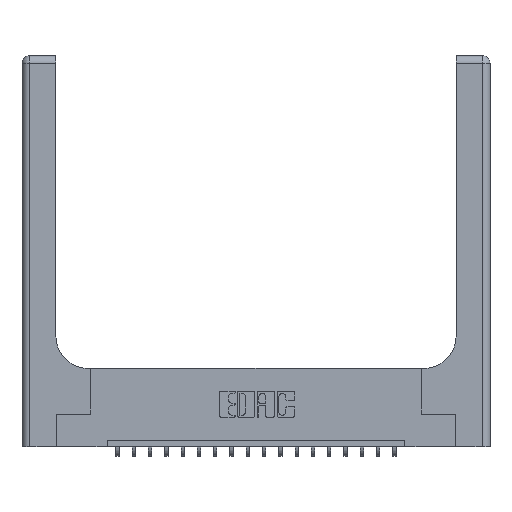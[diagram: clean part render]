
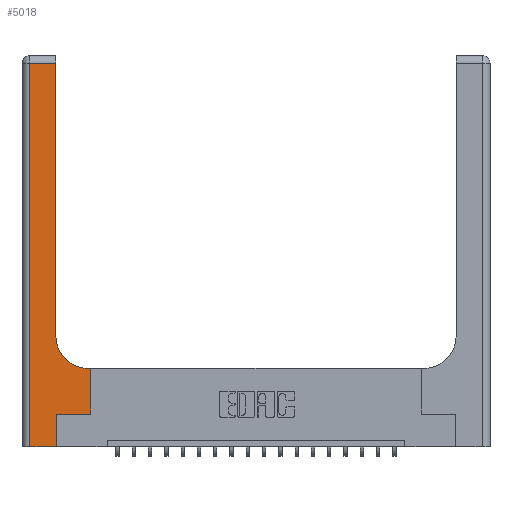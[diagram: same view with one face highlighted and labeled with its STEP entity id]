
A CAD part, top view. The second image highlights one B-rep face of the part: STEP entity #5018.
In plain terms, the highlighted planar face has unit normal (0, 0, 1).
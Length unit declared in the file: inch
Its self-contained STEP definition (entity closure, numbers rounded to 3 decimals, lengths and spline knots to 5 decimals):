
#556 = VERTEX_POINT ( 'NONE', #9216 ) ;
#884 = VERTEX_POINT ( 'NONE', #16140 ) ;
#914 = CARTESIAN_POINT ( 'NONE',  ( 0.528, 0.25, 0.37 ) ) ;
#1122 = LINE ( 'NONE', #17620, #4291 ) ;
#1272 = CARTESIAN_POINT ( 'NONE',  ( 0.51, 0.85, 0.37 ) ) ;
#1273 = ORIENTED_EDGE ( 'NONE', *, *, #6893, .T. ) ;
#1437 = CARTESIAN_POINT ( 'NONE',  ( 0.265, 0.25, 0.37 ) ) ;
#1882 = EDGE_CURVE ( 'NONE', #2824, #1946, #1122, .T. ) ;
#1936 = CARTESIAN_POINT ( 'NONE',  ( 0.265, 0., 0.37 ) ) ;
#1946 = VERTEX_POINT ( 'NONE', #18594 ) ;
#2226 = ORIENTED_EDGE ( 'NONE', *, *, #4807, .T. ) ;
#2437 = CARTESIAN_POINT ( 'NONE',  ( 0.06, 2.94, 0.37 ) ) ;
#2505 = EDGE_CURVE ( 'NONE', #884, #556, #6919, .T. ) ;
#2533 = EDGE_CURVE ( 'NONE', #2787, #11982, #18445, .T. ) ;
#2642 = ORIENTED_EDGE ( 'NONE', *, *, #5450, .T. ) ;
#2787 = VERTEX_POINT ( 'NONE', #7012 ) ;
#2809 = VECTOR ( 'NONE', #9410, 39.37008 ) ;
#2824 = VERTEX_POINT ( 'NONE', #914 ) ;
#2850 = DIRECTION ( 'NONE',  ( 1., 0., 0. ) ) ;
#2891 = DIRECTION ( 'NONE',  ( 1., 0., 0. ) ) ;
#2896 = CARTESIAN_POINT ( 'NONE',  ( 0.51, 0.6, 0.37 ) ) ;
#3967 = LINE ( 'NONE', #1936, #16065 ) ;
#4291 = VECTOR ( 'NONE', #9397, 39.37008 ) ;
#4752 = VECTOR ( 'NONE', #15321, 39.37008 ) ;
#4807 = EDGE_CURVE ( 'NONE', #12909, #2824, #18921, .T. ) ;
#4899 = ORIENTED_EDGE ( 'NONE', *, *, #2533, .T. ) ;
#4968 = PLANE ( 'NONE',  #11999 ) ;
#4972 = ORIENTED_EDGE ( 'NONE', *, *, #2505, .T. ) ;
#5018 = ADVANCED_FACE ( 'NONE', ( #14708 ), #4968, .F. ) ;
#5150 = CARTESIAN_POINT ( 'NONE',  ( 0.26, 2.94, 0.37 ) ) ;
#5159 = EDGE_CURVE ( 'NONE', #9615, #884, #5220, .T. ) ;
#5220 = LINE ( 'NONE', #10884, #4752 ) ;
#5450 = EDGE_CURVE ( 'NONE', #1946, #14128, #11665, .T. ) ;
#6278 = DIRECTION ( 'NONE',  ( 1., 0., 0. ) ) ;
#6517 = DIRECTION ( 'NONE',  ( -1., 0., 0. ) ) ;
#6765 = DIRECTION ( 'NONE',  ( -1., 0., 0. ) ) ;
#6893 = EDGE_CURVE ( 'NONE', #556, #12909, #3967, .T. ) ;
#6919 = LINE ( 'NONE', #10885, #7402 ) ;
#7012 = CARTESIAN_POINT ( 'NONE',  ( 0.26, 0.85, 0.37 ) ) ;
#7402 = VECTOR ( 'NONE', #6278, 39.37008 ) ;
#9216 = CARTESIAN_POINT ( 'NONE',  ( 0.265, 0., 0.37 ) ) ;
#9340 = CARTESIAN_POINT ( 'NONE',  ( 0.26, 3., 0.37 ) ) ;
#9397 = DIRECTION ( 'NONE',  ( 0., 1., 0. ) ) ;
#9410 = DIRECTION ( 'NONE',  ( 0., 1., 0. ) ) ;
#9615 = VERTEX_POINT ( 'NONE', #2437 ) ;
#10002 = DIRECTION ( 'NONE',  ( -1., 0., 0. ) ) ;
#10538 = CARTESIAN_POINT ( 'NONE',  ( 0.265, 0.25, 0.37 ) ) ;
#10884 = CARTESIAN_POINT ( 'NONE',  ( 0.06, 3., 0.37 ) ) ;
#10885 = CARTESIAN_POINT ( 'NONE',  ( 0., 0., 0.37 ) ) ;
#11169 = ORIENTED_EDGE ( 'NONE', *, *, #13569, .T. ) ;
#11474 = CARTESIAN_POINT ( 'NONE',  ( 0.26, 0.6, 0.37 ) ) ;
#11665 = LINE ( 'NONE', #11474, #19131 ) ;
#11691 = VECTOR ( 'NONE', #6765, 39.37008 ) ;
#11982 = VERTEX_POINT ( 'NONE', #5150 ) ;
#11999 = AXIS2_PLACEMENT_3D ( 'NONE', #18503, #15561, #6517 ) ;
#12019 = DIRECTION ( 'NONE',  ( 0., 0., -1. ) ) ;
#12652 = ORIENTED_EDGE ( 'NONE', *, *, #1882, .T. ) ;
#12909 = VERTEX_POINT ( 'NONE', #1437 ) ;
#13569 = EDGE_CURVE ( 'NONE', #14128, #2787, #15926, .T. ) ;
#14128 = VERTEX_POINT ( 'NONE', #2896 ) ;
#14708 = FACE_OUTER_BOUND ( 'NONE', #18203, .T. ) ;
#15049 = EDGE_CURVE ( 'NONE', #11982, #9615, #16143, .T. ) ;
#15292 = ORIENTED_EDGE ( 'NONE', *, *, #15049, .T. ) ;
#15321 = DIRECTION ( 'NONE',  ( 0., -1., 0. ) ) ;
#15561 = DIRECTION ( 'NONE',  ( 0., 0., -1. ) ) ;
#15926 = CIRCLE ( 'NONE', #17598, 0.25 ) ;
#16065 = VECTOR ( 'NONE', #18585, 39.37008 ) ;
#16140 = CARTESIAN_POINT ( 'NONE',  ( 0.06, 0., 0.37 ) ) ;
#16143 = LINE ( 'NONE', #17298, #11691 ) ;
#17298 = CARTESIAN_POINT ( 'NONE',  ( 0., 2.94, 0.37 ) ) ;
#17598 = AXIS2_PLACEMENT_3D ( 'NONE', #1272, #12019, #2850 ) ;
#17620 = CARTESIAN_POINT ( 'NONE',  ( 0.528, 0.25, 0.37 ) ) ;
#17996 = VECTOR ( 'NONE', #2891, 39.37008 ) ;
#18203 = EDGE_LOOP ( 'NONE', ( #4899, #15292, #19444, #4972, #1273, #2226, #12652, #2642, #11169 ) ) ;
#18445 = LINE ( 'NONE', #9340, #2809 ) ;
#18503 = CARTESIAN_POINT ( 'NONE',  ( 0., 3., 0.37 ) ) ;
#18585 = DIRECTION ( 'NONE',  ( 0., 1., 0. ) ) ;
#18594 = CARTESIAN_POINT ( 'NONE',  ( 0.528, 0.6, 0.37 ) ) ;
#18921 = LINE ( 'NONE', #10538, #17996 ) ;
#19131 = VECTOR ( 'NONE', #10002, 39.37008 ) ;
#19444 = ORIENTED_EDGE ( 'NONE', *, *, #5159, .T. ) ;
